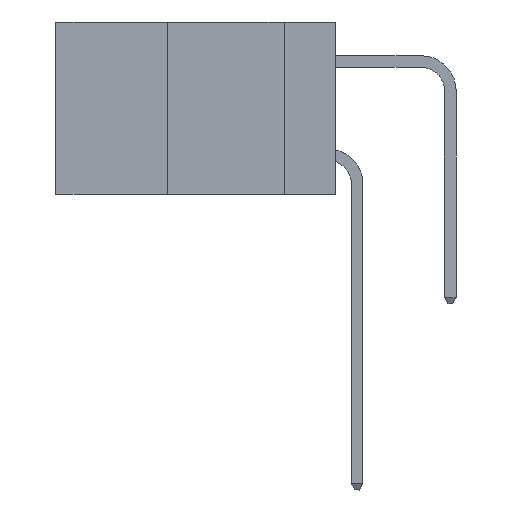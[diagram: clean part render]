
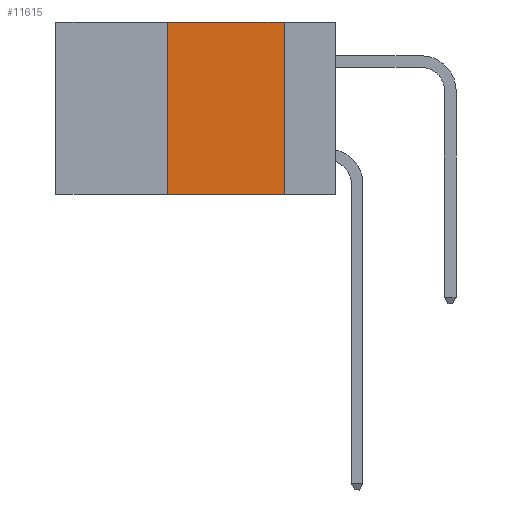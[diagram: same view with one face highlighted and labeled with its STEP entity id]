
A CAD part, left-side view. The second image highlights one B-rep face of the part: STEP entity #11615.
In plain terms, the highlighted planar face has unit normal (-1, 0, 0).
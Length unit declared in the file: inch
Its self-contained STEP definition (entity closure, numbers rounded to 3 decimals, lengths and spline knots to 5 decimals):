
#107 = AXIS2_PLACEMENT_3D ( 'NONE', #10652, #499, #14301 ) ;
#499 = DIRECTION ( 'NONE',  ( 1., 0., 0. ) ) ;
#1043 = DIRECTION ( 'NONE',  ( 0., -1., 0. ) ) ;
#2242 = CARTESIAN_POINT ( 'NONE',  ( 0., 0.11, -0.37 ) ) ;
#3227 = PLANE ( 'NONE',  #107 ) ;
#3426 = DIRECTION ( 'NONE',  ( 0., -1., 0. ) ) ;
#3450 = LINE ( 'NONE', #16251, #5039 ) ;
#3582 = VERTEX_POINT ( 'NONE', #14882 ) ;
#3802 = EDGE_CURVE ( 'NONE', #5910, #11395, #9408, .T. ) ;
#3858 = LINE ( 'NONE', #8887, #6869 ) ;
#3961 = CARTESIAN_POINT ( 'NONE',  ( 0., 0.36, -0.37 ) ) ;
#4158 = ORIENTED_EDGE ( 'NONE', *, *, #6410, .F. ) ;
#5039 = VECTOR ( 'NONE', #1043, 39.37008 ) ;
#5882 = CARTESIAN_POINT ( 'NONE',  ( 0., 0.11, 0. ) ) ;
#5910 = VERTEX_POINT ( 'NONE', #5882 ) ;
#6410 = EDGE_CURVE ( 'NONE', #3582, #5910, #3450, .T. ) ;
#6593 = EDGE_CURVE ( 'NONE', #13323, #3582, #3858, .T. ) ;
#6744 = VECTOR ( 'NONE', #13405, 39.37008 ) ;
#6869 = VECTOR ( 'NONE', #13939, 39.37008 ) ;
#6886 = EDGE_CURVE ( 'NONE', #13323, #11395, #14746, .T. ) ;
#7369 = CARTESIAN_POINT ( 'NONE',  ( 0., 0.6, -0.37 ) ) ;
#8887 = CARTESIAN_POINT ( 'NONE',  ( 0., 0.36, 0. ) ) ;
#9408 = LINE ( 'NONE', #10902, #6744 ) ;
#9856 = ORIENTED_EDGE ( 'NONE', *, *, #6593, .F. ) ;
#10652 = CARTESIAN_POINT ( 'NONE',  ( 0., 0.6, 0. ) ) ;
#10902 = CARTESIAN_POINT ( 'NONE',  ( 0., 0.11, 0. ) ) ;
#11395 = VERTEX_POINT ( 'NONE', #2242 ) ;
#11481 = EDGE_LOOP ( 'NONE', ( #11945, #4158, #9856, #14324 ) ) ;
#11615 = ADVANCED_FACE ( 'NONE', ( #14544 ), #3227, .F. ) ;
#11945 = ORIENTED_EDGE ( 'NONE', *, *, #3802, .F. ) ;
#13323 = VERTEX_POINT ( 'NONE', #3961 ) ;
#13405 = DIRECTION ( 'NONE',  ( 0., 0., -1. ) ) ;
#13939 = DIRECTION ( 'NONE',  ( 0., 0., 1. ) ) ;
#14301 = DIRECTION ( 'NONE',  ( 0., 0., -1. ) ) ;
#14324 = ORIENTED_EDGE ( 'NONE', *, *, #6886, .T. ) ;
#14544 = FACE_OUTER_BOUND ( 'NONE', #11481, .T. ) ;
#14547 = VECTOR ( 'NONE', #3426, 39.37008 ) ;
#14746 = LINE ( 'NONE', #7369, #14547 ) ;
#14882 = CARTESIAN_POINT ( 'NONE',  ( 0., 0.36, 0. ) ) ;
#16251 = CARTESIAN_POINT ( 'NONE',  ( 0., 0.6, 0. ) ) ;
